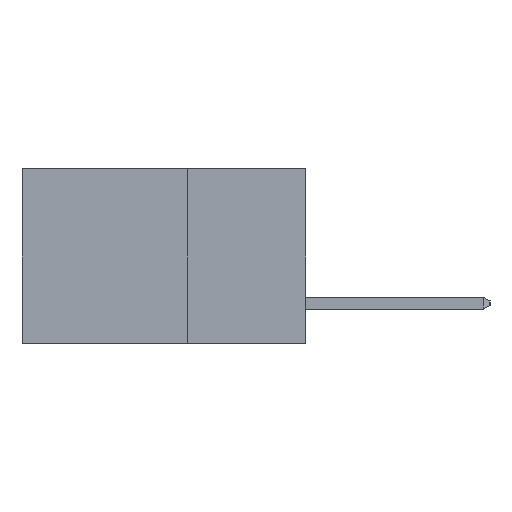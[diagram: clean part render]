
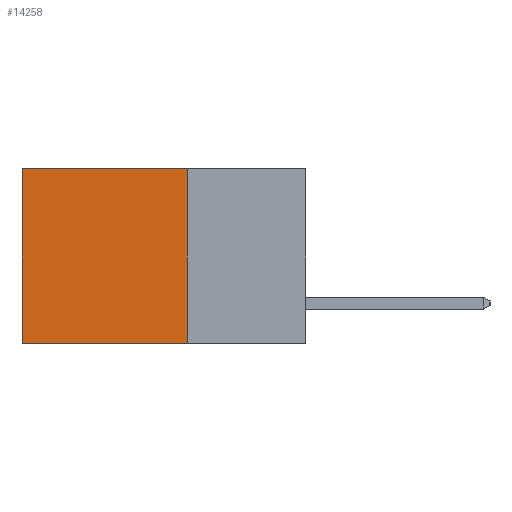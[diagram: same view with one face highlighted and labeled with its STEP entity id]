
A CAD part, left-side view. The second image highlights one B-rep face of the part: STEP entity #14258.
In plain terms, the highlighted planar face has unit normal (-1, 0, 0).
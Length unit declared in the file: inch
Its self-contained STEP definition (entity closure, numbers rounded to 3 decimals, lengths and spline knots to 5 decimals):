
#1962 = ORIENTED_EDGE ( 'NONE', *, *, #13904, .T. ) ;
#3518 = FACE_OUTER_BOUND ( 'NONE', #11821, .T. ) ;
#4516 = VERTEX_POINT ( 'NONE', #11224 ) ;
#5478 = CARTESIAN_POINT ( 'NONE',  ( 0.2615, 0.25, -0.37 ) ) ;
#6227 = CARTESIAN_POINT ( 'NONE',  ( 0.2615, 0.6, -0.37 ) ) ;
#7013 = EDGE_CURVE ( 'NONE', #8066, #18246, #15428, .T. ) ;
#7063 = VECTOR ( 'NONE', #11409, 39.37008 ) ;
#7143 = DIRECTION ( 'NONE',  ( 0., 0., -1. ) ) ;
#8066 = VERTEX_POINT ( 'NONE', #5478 ) ;
#8575 = EDGE_CURVE ( 'NONE', #14372, #8066, #23937, .T. ) ;
#9343 = CARTESIAN_POINT ( 'NONE',  ( 0.2615, 0.25, 0. ) ) ;
#9408 = ORIENTED_EDGE ( 'NONE', *, *, #7013, .F. ) ;
#10405 = PLANE ( 'NONE',  #20505 ) ;
#11224 = CARTESIAN_POINT ( 'NONE',  ( 0.2615, 0.6, 0. ) ) ;
#11409 = DIRECTION ( 'NONE',  ( 0., 1., 0. ) ) ;
#11821 = EDGE_LOOP ( 'NONE', ( #20141, #9408, #23142, #1962 ) ) ;
#12372 = CARTESIAN_POINT ( 'NONE',  ( 0.2615, 0.25, -0.37 ) ) ;
#12459 = DIRECTION ( 'NONE',  ( 0., 0., -1. ) ) ;
#12712 = CARTESIAN_POINT ( 'NONE',  ( 0.2615, 0.25, 0. ) ) ;
#13134 = LINE ( 'NONE', #9343, #7063 ) ;
#13904 = EDGE_CURVE ( 'NONE', #14372, #4516, #13134, .T. ) ;
#14258 = ADVANCED_FACE ( 'NONE', ( #3518 ), #10405, .F. ) ;
#14372 = VERTEX_POINT ( 'NONE', #12712 ) ;
#15428 = LINE ( 'NONE', #17773, #20029 ) ;
#17644 = DIRECTION ( 'NONE',  ( 0., 1., 0. ) ) ;
#17773 = CARTESIAN_POINT ( 'NONE',  ( 0.2615, 0.25, -0.37 ) ) ;
#17889 = EDGE_CURVE ( 'NONE', #4516, #18246, #24773, .T. ) ;
#18246 = VERTEX_POINT ( 'NONE', #6227 ) ;
#18797 = VECTOR ( 'NONE', #20206, 39.37008 ) ;
#19016 = VECTOR ( 'NONE', #7143, 39.37008 ) ;
#20029 = VECTOR ( 'NONE', #17644, 39.37008 ) ;
#20141 = ORIENTED_EDGE ( 'NONE', *, *, #17889, .T. ) ;
#20206 = DIRECTION ( 'NONE',  ( 0., 0., -1. ) ) ;
#20505 = AXIS2_PLACEMENT_3D ( 'NONE', #12372, #24223, #12459 ) ;
#20881 = CARTESIAN_POINT ( 'NONE',  ( 0.2615, 0.25, -0.37 ) ) ;
#23071 = CARTESIAN_POINT ( 'NONE',  ( 0.2615, 0.6, -0.37 ) ) ;
#23142 = ORIENTED_EDGE ( 'NONE', *, *, #8575, .F. ) ;
#23937 = LINE ( 'NONE', #20881, #18797 ) ;
#24223 = DIRECTION ( 'NONE',  ( 1., 0., 0. ) ) ;
#24773 = LINE ( 'NONE', #23071, #19016 ) ;
